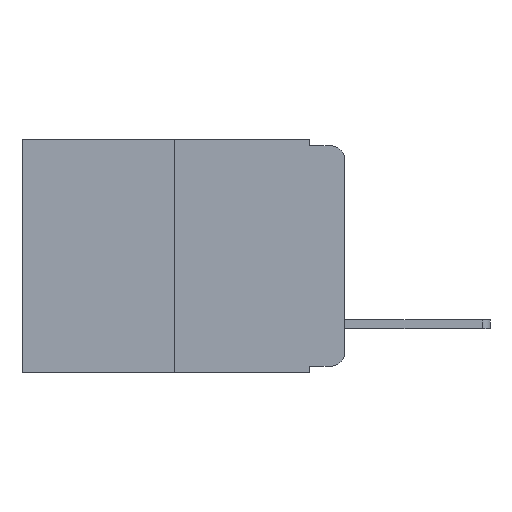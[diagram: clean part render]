
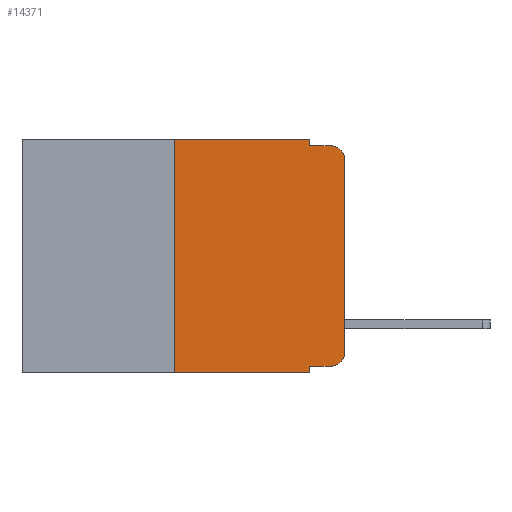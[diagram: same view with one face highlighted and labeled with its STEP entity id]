
A CAD part, left-side view. The second image highlights one B-rep face of the part: STEP entity #14371.
In plain terms, the highlighted planar face has unit normal (-1, 0, 0).
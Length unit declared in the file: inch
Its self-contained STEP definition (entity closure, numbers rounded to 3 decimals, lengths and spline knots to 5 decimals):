
#47 = CARTESIAN_POINT ( 'NONE',  ( 0., 0.051, -0.333 ) ) ;
#78 = DIRECTION ( 'NONE',  ( 0., -1., 0. ) ) ;
#915 = ORIENTED_EDGE ( 'NONE', *, *, #13782, .T. ) ;
#1322 = EDGE_CURVE ( 'NONE', #6679, #12473, #3140, .T. ) ;
#1401 = LINE ( 'NONE', #47, #12990 ) ;
#1485 = CARTESIAN_POINT ( 'NONE',  ( 0., 0.051, -0.01 ) ) ;
#1520 = ORIENTED_EDGE ( 'NONE', *, *, #10856, .T. ) ;
#1549 = CARTESIAN_POINT ( 'NONE',  ( 0., 0.02, -0.333 ) ) ;
#1833 = ORIENTED_EDGE ( 'NONE', *, *, #1998, .F. ) ;
#1983 = CARTESIAN_POINT ( 'NONE',  ( 0., 0., -0.03 ) ) ;
#1998 = EDGE_CURVE ( 'NONE', #13457, #6057, #14436, .T. ) ;
#2154 = ORIENTED_EDGE ( 'NONE', *, *, #13617, .T. ) ;
#2309 = CARTESIAN_POINT ( 'NONE',  ( 0., 0.473, 0. ) ) ;
#2344 = EDGE_LOOP ( 'NONE', ( #915, #1520, #8517, #14416, #1833, #10452, #6889, #3706, #5640, #2154 ) ) ;
#2454 = VERTEX_POINT ( 'NONE', #1983 ) ;
#2478 = CARTESIAN_POINT ( 'NONE',  ( 0., 0.051, -0.01 ) ) ;
#2492 = PLANE ( 'NONE',  #10215 ) ;
#2794 = DIRECTION ( 'NONE',  ( -1., 0., 0. ) ) ;
#3119 = LINE ( 'NONE', #5851, #8761 ) ;
#3140 = LINE ( 'NONE', #7885, #11766 ) ;
#3395 = CARTESIAN_POINT ( 'NONE',  ( 0., 0.25, 0. ) ) ;
#3521 = DIRECTION ( 'NONE',  ( 0., 0., 1. ) ) ;
#3571 = EDGE_CURVE ( 'NONE', #7612, #13457, #13587, .T. ) ;
#3667 = FACE_OUTER_BOUND ( 'NONE', #2344, .T. ) ;
#3706 = ORIENTED_EDGE ( 'NONE', *, *, #1322, .F. ) ;
#4174 = VERTEX_POINT ( 'NONE', #1485 ) ;
#4648 = DIRECTION ( 'NONE',  ( 0., 0., -1. ) ) ;
#4747 = CARTESIAN_POINT ( 'NONE',  ( 0., 0.473, 0. ) ) ;
#4935 = CIRCLE ( 'NONE', #10308, 0.02 ) ;
#5541 = DIRECTION ( 'NONE',  ( -1., 0., 0. ) ) ;
#5575 = VECTOR ( 'NONE', #9905, 39.37008 ) ;
#5640 = ORIENTED_EDGE ( 'NONE', *, *, #14301, .T. ) ;
#5851 = CARTESIAN_POINT ( 'NONE',  ( 0., 0.051, 0. ) ) ;
#5862 = DIRECTION ( 'NONE',  ( 0., 0., -1. ) ) ;
#6057 = VERTEX_POINT ( 'NONE', #14193 ) ;
#6064 = CARTESIAN_POINT ( 'NONE',  ( 0., 0.25, 0. ) ) ;
#6679 = VERTEX_POINT ( 'NONE', #11972 ) ;
#6831 = VECTOR ( 'NONE', #11496, 39.37008 ) ;
#6889 = ORIENTED_EDGE ( 'NONE', *, *, #7345, .T. ) ;
#7038 = EDGE_CURVE ( 'NONE', #6057, #4174, #3119, .T. ) ;
#7042 = LINE ( 'NONE', #2478, #12690 ) ;
#7345 = EDGE_CURVE ( 'NONE', #7612, #12473, #7853, .T. ) ;
#7612 = VERTEX_POINT ( 'NONE', #9055 ) ;
#7687 = VERTEX_POINT ( 'NONE', #12583 ) ;
#7853 = LINE ( 'NONE', #8606, #10501 ) ;
#7885 = CARTESIAN_POINT ( 'NONE',  ( 0., 0.051, 0. ) ) ;
#7990 = DIRECTION ( 'NONE',  ( 0., -1., 0. ) ) ;
#8517 = ORIENTED_EDGE ( 'NONE', *, *, #10084, .F. ) ;
#8606 = CARTESIAN_POINT ( 'NONE',  ( 0., 0.473, -0.343 ) ) ;
#8761 = VECTOR ( 'NONE', #9226, 39.37008 ) ;
#9055 = CARTESIAN_POINT ( 'NONE',  ( 0., 0.25, -0.343 ) ) ;
#9226 = DIRECTION ( 'NONE',  ( 0., 0., -1. ) ) ;
#9251 = CARTESIAN_POINT ( 'NONE',  ( 0., 0., 0. ) ) ;
#9528 = CARTESIAN_POINT ( 'NONE',  ( 0., 0.02, -0.03 ) ) ;
#9905 = DIRECTION ( 'NONE',  ( 0., -1., 0. ) ) ;
#10084 = EDGE_CURVE ( 'NONE', #4174, #11906, #7042, .T. ) ;
#10215 = AXIS2_PLACEMENT_3D ( 'NONE', #4747, #12607, #5862 ) ;
#10308 = AXIS2_PLACEMENT_3D ( 'NONE', #12290, #5541, #13374 ) ;
#10452 = ORIENTED_EDGE ( 'NONE', *, *, #3571, .F. ) ;
#10501 = VECTOR ( 'NONE', #12008, 39.37008 ) ;
#10663 = DIRECTION ( 'NONE',  ( 0., 0., -1. ) ) ;
#10856 = EDGE_CURVE ( 'NONE', #2454, #11906, #12009, .T. ) ;
#11006 = VECTOR ( 'NONE', #3521, 39.37008 ) ;
#11496 = DIRECTION ( 'NONE',  ( 0., 0., 1. ) ) ;
#11766 = VECTOR ( 'NONE', #4648, 39.37008 ) ;
#11906 = VERTEX_POINT ( 'NONE', #12596 ) ;
#11972 = CARTESIAN_POINT ( 'NONE',  ( 0., 0.051, -0.333 ) ) ;
#12008 = DIRECTION ( 'NONE',  ( 0., -1., 0. ) ) ;
#12009 = CIRCLE ( 'NONE', #13777, 0.02 ) ;
#12154 = LINE ( 'NONE', #9251, #6831 ) ;
#12290 = CARTESIAN_POINT ( 'NONE',  ( 0., 0.02, -0.313 ) ) ;
#12473 = VERTEX_POINT ( 'NONE', #13783 ) ;
#12583 = CARTESIAN_POINT ( 'NONE',  ( 0., 0., -0.313 ) ) ;
#12596 = CARTESIAN_POINT ( 'NONE',  ( 0., 0.02, -0.01 ) ) ;
#12607 = DIRECTION ( 'NONE',  ( 1., 0., 0. ) ) ;
#12690 = VECTOR ( 'NONE', #78, 39.37008 ) ;
#12758 = VERTEX_POINT ( 'NONE', #1549 ) ;
#12990 = VECTOR ( 'NONE', #7990, 39.37008 ) ;
#13374 = DIRECTION ( 'NONE',  ( 0., 0., -1. ) ) ;
#13457 = VERTEX_POINT ( 'NONE', #6064 ) ;
#13587 = LINE ( 'NONE', #3395, #11006 ) ;
#13617 = EDGE_CURVE ( 'NONE', #12758, #7687, #4935, .T. ) ;
#13777 = AXIS2_PLACEMENT_3D ( 'NONE', #9528, #2794, #10663 ) ;
#13782 = EDGE_CURVE ( 'NONE', #7687, #2454, #12154, .T. ) ;
#13783 = CARTESIAN_POINT ( 'NONE',  ( 0., 0.051, -0.343 ) ) ;
#14193 = CARTESIAN_POINT ( 'NONE',  ( 0., 0.051, 0. ) ) ;
#14301 = EDGE_CURVE ( 'NONE', #6679, #12758, #1401, .T. ) ;
#14371 = ADVANCED_FACE ( 'NONE', ( #3667 ), #2492, .F. ) ;
#14416 = ORIENTED_EDGE ( 'NONE', *, *, #7038, .F. ) ;
#14436 = LINE ( 'NONE', #2309, #5575 ) ;
